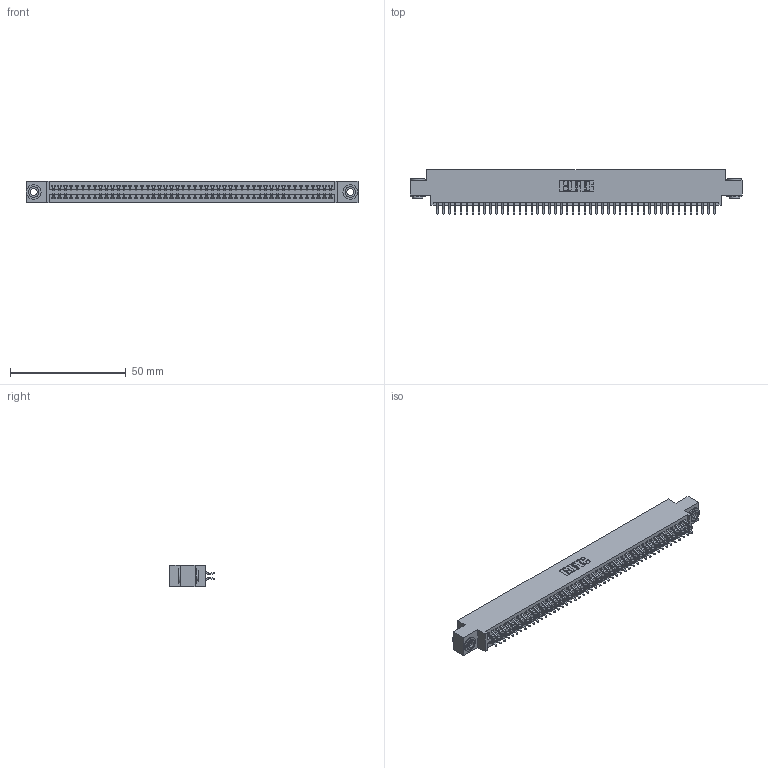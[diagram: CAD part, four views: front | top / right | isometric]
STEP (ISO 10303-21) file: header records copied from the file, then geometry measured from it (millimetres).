
FILE_DESCRIPTION (( 'STEP AP203' ), '1' );
FILE_NAME ('345-096-556-803.STEP', '2019-11-02T09:01:59', ( '' ), ( '' ), 'SwSTEP 2.0', 'SolidWorks 2016', '' );
FILE_SCHEMA (( 'CONFIG_CONTROL_DESIGN' ));
Length unit declared in the file: inch
Products named in the file (4): 345 Part_0.170 Offset - 0.156 Dia-TH; 345-096-556-803; 345-250-002_345-250-002-102; 345-292-001_556 Tail
Assembly tree (99 placements, depth 2):
  345-096-556-803
    345 Part_0.170 Offset - 0.156 Dia-TH
    345-292-001_556 Tail  x96
    345-250-002_345-250-002-102  x2
Bounding box: 143.13 x 19.24 x 9.4 mm (x, y, z)
Volume: 13861.6 mm3; surface area: 20870.3 mm2
Topology: 99 solids, 99 shells, 5544 faces, 16461 edges, 10842 vertices
Faces by surface type: plane 3646, cylinder 1890, cone 8
Entity records: 37856 total; most frequent: CARTESIAN_POINT 6331, ORIENTED_EDGE 6246, DIRECTION 5593, EDGE_CURVE 3123, LINE 2767, VECTOR 2767, VERTEX_POINT 2078, AXIS2_PLACEMENT_3D 1413
